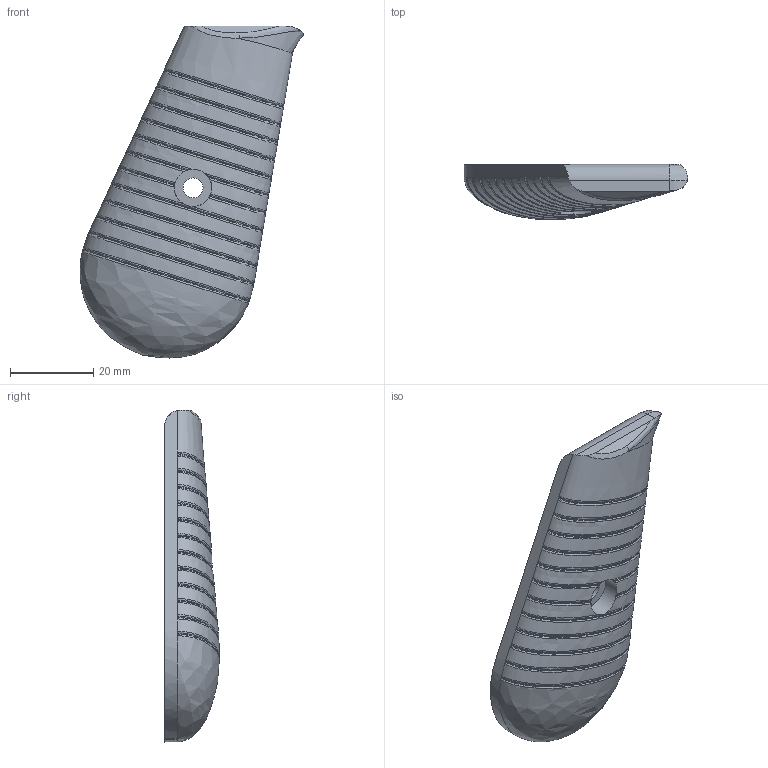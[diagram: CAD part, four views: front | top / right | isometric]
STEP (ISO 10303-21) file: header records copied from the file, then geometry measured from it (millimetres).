
FILE_DESCRIPTION(/* description */ (''),/* implementation_level */ '2;1');
FILE_NAME(/* name */ 'Right Grip Plate.step',/* time_stamp */ '2021-09-21T09:20:24-04:00',/* author */ (''),/* organization */ (''),/* preprocessor_version */ 'ST-DEVELOPER v18.1',/* originating_system */ 'Autodesk Translation Framework v10.10.0.1391',/* authorisation */ '');
FILE_SCHEMA (('AUTOMOTIVE_DESIGN { 1 0 10303 214 3 1 1 }'));
Length unit declared in the file: millimetre
Products named in the file (1): Right Grip Plate
Bounding box: 53.86 x 13.19 x 79.86 mm (x, y, z)
Volume: 25639 mm3; surface area: 7382.5 mm2
Topology: 1 solids, 1 shells, 127 faces, 322 edges, 198 vertices
Faces by surface type: bspline 80, plane 38, cylinder 9
Full cylindrical faces by diameter (mm): 4.8 x1, 9 x1
Entity records: 21732 total; most frequent: CARTESIAN_POINT 19302, ORIENTED_EDGE 644, EDGE_CURVE 322, DIRECTION 235, B_SPLINE_CURVE_WITH_KNOTS 218, VERTEX_POINT 198, EDGE_LOOP 130, FACE_OUTER_BOUND 127
